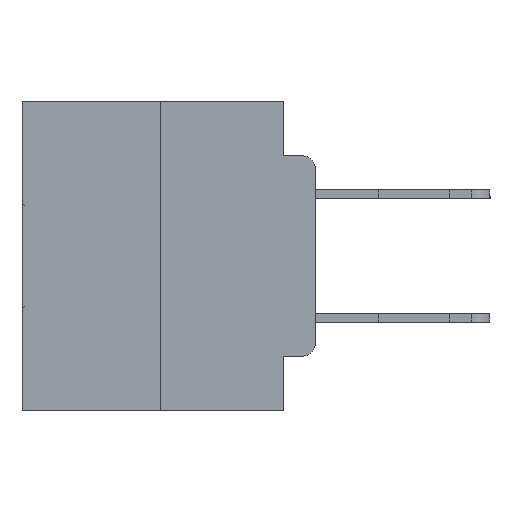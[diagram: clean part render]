
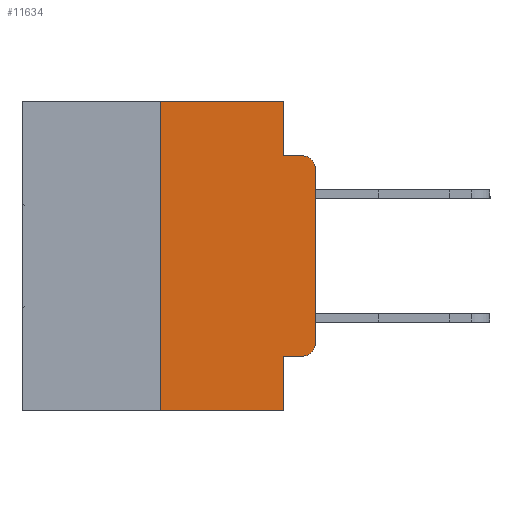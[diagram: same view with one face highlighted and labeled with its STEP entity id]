
A CAD part, left-side view. The second image highlights one B-rep face of the part: STEP entity #11634.
In plain terms, the highlighted planar face has unit normal (-1, 0, 0).
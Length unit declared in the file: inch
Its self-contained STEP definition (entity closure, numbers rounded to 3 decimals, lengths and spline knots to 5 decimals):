
#192 = AXIS2_PLACEMENT_3D ( 'NONE', #457, #17320, #2944 ) ;
#457 = CARTESIAN_POINT ( 'NONE',  ( 0., 0.02, -0.1085 ) ) ;
#533 = PLANE ( 'NONE',  #12325 ) ;
#1426 = VECTOR ( 'NONE', #17007, 39.37008 ) ;
#1572 = CARTESIAN_POINT ( 'NONE',  ( 0., 0.051, 0. ) ) ;
#2501 = CARTESIAN_POINT ( 'NONE',  ( 0., 0., -0.1085 ) ) ;
#2895 = ORIENTED_EDGE ( 'NONE', *, *, #24018, .T. ) ;
#2907 = VERTEX_POINT ( 'NONE', #28441 ) ;
#2944 = DIRECTION ( 'NONE',  ( 0., 0., -1. ) ) ;
#3270 = EDGE_CURVE ( 'NONE', #2907, #13893, #15118, .T. ) ;
#3692 = EDGE_CURVE ( 'NONE', #13747, #4824, #10213, .T. ) ;
#4152 = VERTEX_POINT ( 'NONE', #9860 ) ;
#4824 = VERTEX_POINT ( 'NONE', #11954 ) ;
#5185 = ORIENTED_EDGE ( 'NONE', *, *, #24794, .F. ) ;
#5878 = ORIENTED_EDGE ( 'NONE', *, *, #29331, .F. ) ;
#7011 = CARTESIAN_POINT ( 'NONE',  ( 0., 0.25, -0.5 ) ) ;
#7131 = ORIENTED_EDGE ( 'NONE', *, *, #13901, .T. ) ;
#7349 = VECTOR ( 'NONE', #13074, 39.37008 ) ;
#7546 = CARTESIAN_POINT ( 'NONE',  ( 0., 0., -0.3915 ) ) ;
#7730 = CARTESIAN_POINT ( 'NONE',  ( 0., 0.051, -0.4115 ) ) ;
#7822 = DIRECTION ( 'NONE',  ( 0., 0., -1. ) ) ;
#7833 = CIRCLE ( 'NONE', #192, 0.02 ) ;
#7999 = VECTOR ( 'NONE', #18324, 39.37008 ) ;
#8096 = LINE ( 'NONE', #17877, #7349 ) ;
#8172 = FACE_OUTER_BOUND ( 'NONE', #8864, .T. ) ;
#8566 = LINE ( 'NONE', #26193, #1426 ) ;
#8864 = EDGE_LOOP ( 'NONE', ( #19631, #7131, #5185, #5878, #22663, #26982, #14656, #10261, #2895, #14771 ) ) ;
#9860 = CARTESIAN_POINT ( 'NONE',  ( 0., 0.02, -0.0885 ) ) ;
#10125 = DIRECTION ( 'NONE',  ( 0., -1., 0. ) ) ;
#10213 = LINE ( 'NONE', #12742, #27355 ) ;
#10261 = ORIENTED_EDGE ( 'NONE', *, *, #18659, .F. ) ;
#11071 = CARTESIAN_POINT ( 'NONE',  ( 0., 0.02, -0.3915 ) ) ;
#11205 = VECTOR ( 'NONE', #29874, 39.37008 ) ;
#11376 = CARTESIAN_POINT ( 'NONE',  ( 0., 0.051, 0. ) ) ;
#11634 = ADVANCED_FACE ( 'NONE', ( #8172 ), #533, .F. ) ;
#11889 = LINE ( 'NONE', #7730, #23611 ) ;
#11954 = CARTESIAN_POINT ( 'NONE',  ( 0., 0.051, -0.5 ) ) ;
#12305 = CARTESIAN_POINT ( 'NONE',  ( 0., 0.473, 0. ) ) ;
#12325 = AXIS2_PLACEMENT_3D ( 'NONE', #26456, #22015, #7822 ) ;
#12717 = LINE ( 'NONE', #11376, #11205 ) ;
#12742 = CARTESIAN_POINT ( 'NONE',  ( 0., 0.473, -0.5 ) ) ;
#12842 = DIRECTION ( 'NONE',  ( 0., -1., 0. ) ) ;
#13074 = DIRECTION ( 'NONE',  ( 0., 0., 1. ) ) ;
#13382 = VERTEX_POINT ( 'NONE', #16986 ) ;
#13461 = DIRECTION ( 'NONE',  ( 0., 0., -1. ) ) ;
#13747 = VERTEX_POINT ( 'NONE', #7011 ) ;
#13844 = EDGE_CURVE ( 'NONE', #13893, #23899, #8566, .T. ) ;
#13893 = VERTEX_POINT ( 'NONE', #7546 ) ;
#13901 = EDGE_CURVE ( 'NONE', #23899, #4152, #7833, .T. ) ;
#14656 = ORIENTED_EDGE ( 'NONE', *, *, #3692, .T. ) ;
#14771 = ORIENTED_EDGE ( 'NONE', *, *, #3270, .T. ) ;
#14864 = CARTESIAN_POINT ( 'NONE',  ( 0., 0.051, 0. ) ) ;
#15118 = CIRCLE ( 'NONE', #16773, 0.02 ) ;
#16444 = LINE ( 'NONE', #12305, #28613 ) ;
#16773 = AXIS2_PLACEMENT_3D ( 'NONE', #11071, #27343, #13461 ) ;
#16986 = CARTESIAN_POINT ( 'NONE',  ( 0., 0.051, -0.4115 ) ) ;
#17007 = DIRECTION ( 'NONE',  ( 0., 0., 1. ) ) ;
#17320 = DIRECTION ( 'NONE',  ( -1., 0., 0. ) ) ;
#17877 = CARTESIAN_POINT ( 'NONE',  ( 0., 0.25, 0. ) ) ;
#18041 = CARTESIAN_POINT ( 'NONE',  ( 0., 0.25, 0. ) ) ;
#18324 = DIRECTION ( 'NONE',  ( 0., 0., -1. ) ) ;
#18659 = EDGE_CURVE ( 'NONE', #13382, #4824, #25964, .T. ) ;
#19631 = ORIENTED_EDGE ( 'NONE', *, *, #13844, .T. ) ;
#20355 = VECTOR ( 'NONE', #26816, 39.37008 ) ;
#21889 = CARTESIAN_POINT ( 'NONE',  ( 0., 0.051, -0.0885 ) ) ;
#22015 = DIRECTION ( 'NONE',  ( 1., 0., 0. ) ) ;
#22062 = VERTEX_POINT ( 'NONE', #14864 ) ;
#22663 = ORIENTED_EDGE ( 'NONE', *, *, #29575, .F. ) ;
#23611 = VECTOR ( 'NONE', #10125, 39.37008 ) ;
#23899 = VERTEX_POINT ( 'NONE', #2501 ) ;
#24018 = EDGE_CURVE ( 'NONE', #13382, #2907, #11889, .T. ) ;
#24661 = VERTEX_POINT ( 'NONE', #21889 ) ;
#24794 = EDGE_CURVE ( 'NONE', #24661, #4152, #26393, .T. ) ;
#25303 = EDGE_CURVE ( 'NONE', #13747, #27713, #8096, .T. ) ;
#25964 = LINE ( 'NONE', #1572, #7999 ) ;
#26193 = CARTESIAN_POINT ( 'NONE',  ( 0., 0., 0. ) ) ;
#26393 = LINE ( 'NONE', #29086, #20355 ) ;
#26456 = CARTESIAN_POINT ( 'NONE',  ( 0., 0.473, 0. ) ) ;
#26816 = DIRECTION ( 'NONE',  ( 0., -1., 0. ) ) ;
#26982 = ORIENTED_EDGE ( 'NONE', *, *, #25303, .F. ) ;
#27343 = DIRECTION ( 'NONE',  ( -1., 0., 0. ) ) ;
#27355 = VECTOR ( 'NONE', #12842, 39.37008 ) ;
#27713 = VERTEX_POINT ( 'NONE', #18041 ) ;
#28441 = CARTESIAN_POINT ( 'NONE',  ( 0., 0.02, -0.4115 ) ) ;
#28500 = DIRECTION ( 'NONE',  ( 0., -1., 0. ) ) ;
#28613 = VECTOR ( 'NONE', #28500, 39.37008 ) ;
#29086 = CARTESIAN_POINT ( 'NONE',  ( 0., 0.051, -0.0885 ) ) ;
#29331 = EDGE_CURVE ( 'NONE', #22062, #24661, #12717, .T. ) ;
#29575 = EDGE_CURVE ( 'NONE', #27713, #22062, #16444, .T. ) ;
#29874 = DIRECTION ( 'NONE',  ( 0., 0., -1. ) ) ;
